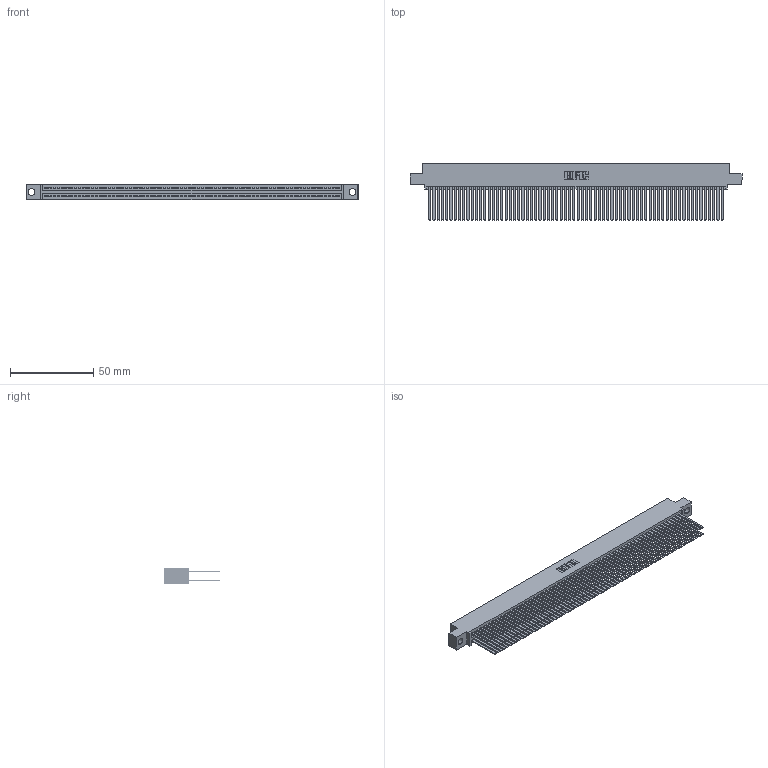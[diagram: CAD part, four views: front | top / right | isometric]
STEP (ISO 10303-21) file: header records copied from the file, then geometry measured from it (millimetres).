
FILE_DESCRIPTION (( 'STEP AP203' ), '1' );
FILE_NAME ('395-140-544-504.STEP', '2021-06-18T04:38:16', ( '' ), ( '' ), 'SwSTEP 2.0', 'SolidWorks 2020', '' );
FILE_SCHEMA (( 'CONFIG_CONTROL_DESIGN' ));
Length unit declared in the file: inch
Products named in the file (3): 345 Part_0.110 Offset - 0.156 Dia-TI; 345-292-001_345-293-144; 395-140-544-504
Assembly tree (141 placements, depth 2):
  395-140-544-504
    345 Part_0.110 Offset - 0.156 Dia-TI
    345-292-001_345-293-144  x140
Bounding box: 199.01 x 33.96 x 9.4 mm (x, y, z)
Volume: 21375.1 mm3; surface area: 37834.7 mm2
Topology: 141 solids, 141 shells, 6304 faces, 18729 edges, 12298 vertices
Faces by surface type: plane 4158, cylinder 2146
Entity records: 51521 total; most frequent: CARTESIAN_POINT 8614, ORIENTED_EDGE 8546, DIRECTION 7557, EDGE_CURVE 4273, LINE 3865, VECTOR 3865, VERTEX_POINT 2846, AXIS2_PLACEMENT_3D 1846
